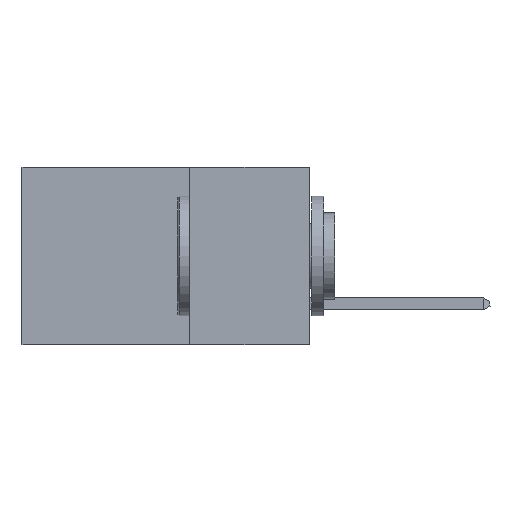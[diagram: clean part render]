
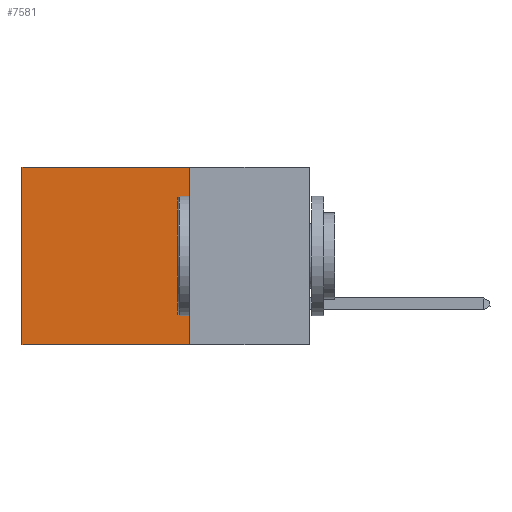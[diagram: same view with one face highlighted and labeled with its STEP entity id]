
A CAD part, left-side view. The second image highlights one B-rep face of the part: STEP entity #7581.
In plain terms, the highlighted planar face has unit normal (-1, 0, 0).
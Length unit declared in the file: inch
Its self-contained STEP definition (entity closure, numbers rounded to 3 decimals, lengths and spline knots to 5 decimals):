
#82 = VECTOR ( 'NONE', #2805, 39.37008 ) ;
#451 = VERTEX_POINT ( 'NONE', #7525 ) ;
#637 = EDGE_CURVE ( 'NONE', #6734, #835, #9340, .T. ) ;
#835 = VERTEX_POINT ( 'NONE', #10612 ) ;
#1844 = CARTESIAN_POINT ( 'NONE',  ( 0.2875, 0.25, 0. ) ) ;
#2805 = DIRECTION ( 'NONE',  ( 0., 0., -1. ) ) ;
#2966 = LINE ( 'NONE', #9189, #9065 ) ;
#3183 = CARTESIAN_POINT ( 'NONE',  ( 0.2875, 0.6, 0. ) ) ;
#3492 = VERTEX_POINT ( 'NONE', #11147 ) ;
#3663 = DIRECTION ( 'NONE',  ( 0., 1., 0. ) ) ;
#3896 = EDGE_CURVE ( 'NONE', #6734, #3492, #2966, .T. ) ;
#4443 = DIRECTION ( 'NONE',  ( 1., 0., 0. ) ) ;
#4655 = ORIENTED_EDGE ( 'NONE', *, *, #6158, .T. ) ;
#4970 = ORIENTED_EDGE ( 'NONE', *, *, #10514, .F. ) ;
#5090 = ORIENTED_EDGE ( 'NONE', *, *, #3896, .F. ) ;
#5116 = ORIENTED_EDGE ( 'NONE', *, *, #637, .T. ) ;
#5222 = VECTOR ( 'NONE', #6598, 39.37008 ) ;
#5311 = PLANE ( 'NONE',  #7797 ) ;
#5410 = CARTESIAN_POINT ( 'NONE',  ( 0.2875, 0.25, 0. ) ) ;
#6158 = EDGE_CURVE ( 'NONE', #835, #451, #9081, .T. ) ;
#6264 = FACE_OUTER_BOUND ( 'NONE', #10759, .T. ) ;
#6598 = DIRECTION ( 'NONE',  ( 0., 1., 0. ) ) ;
#6734 = VERTEX_POINT ( 'NONE', #1844 ) ;
#7125 = CARTESIAN_POINT ( 'NONE',  ( 0.2875, 0.25, 0. ) ) ;
#7322 = LINE ( 'NONE', #7456, #5222 ) ;
#7456 = CARTESIAN_POINT ( 'NONE',  ( 0.2875, 0.25, -0.37 ) ) ;
#7525 = CARTESIAN_POINT ( 'NONE',  ( 0.2875, 0.6, -0.37 ) ) ;
#7581 = ADVANCED_FACE ( 'NONE', ( #6264 ), #5311, .F. ) ;
#7797 = AXIS2_PLACEMENT_3D ( 'NONE', #7125, #4443, #10253 ) ;
#9029 = DIRECTION ( 'NONE',  ( 0., 0., -1. ) ) ;
#9065 = VECTOR ( 'NONE', #9029, 39.37008 ) ;
#9081 = LINE ( 'NONE', #3183, #82 ) ;
#9189 = CARTESIAN_POINT ( 'NONE',  ( 0.2875, 0.25, 0. ) ) ;
#9340 = LINE ( 'NONE', #5410, #11134 ) ;
#10253 = DIRECTION ( 'NONE',  ( 0., 0., -1. ) ) ;
#10514 = EDGE_CURVE ( 'NONE', #3492, #451, #7322, .T. ) ;
#10612 = CARTESIAN_POINT ( 'NONE',  ( 0.2875, 0.6, 0. ) ) ;
#10759 = EDGE_LOOP ( 'NONE', ( #4655, #4970, #5090, #5116 ) ) ;
#11134 = VECTOR ( 'NONE', #3663, 39.37008 ) ;
#11147 = CARTESIAN_POINT ( 'NONE',  ( 0.2875, 0.25, -0.37 ) ) ;
